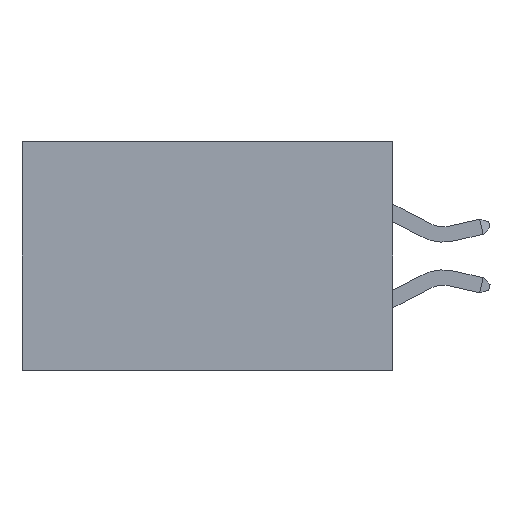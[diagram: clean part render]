
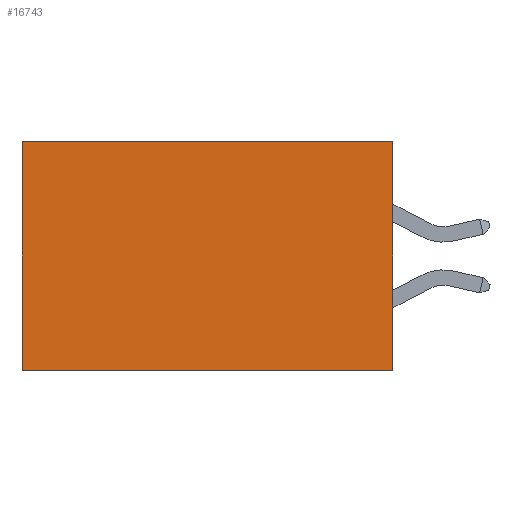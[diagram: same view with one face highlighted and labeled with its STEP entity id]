
A CAD part, left-side view. The second image highlights one B-rep face of the part: STEP entity #16743.
In plain terms, the highlighted planar face has unit normal (-1, 0, 0).
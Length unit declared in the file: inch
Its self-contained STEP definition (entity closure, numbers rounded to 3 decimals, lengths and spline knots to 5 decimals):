
#55 = EDGE_CURVE ( 'NONE', #21798, #2846, #15903, .T. ) ;
#849 = CARTESIAN_POINT ( 'NONE',  ( 0.2875, 0., 0. ) ) ;
#1491 = DIRECTION ( 'NONE',  ( 0., 1., 0. ) ) ;
#2163 = LINE ( 'NONE', #11812, #12779 ) ;
#2846 = VERTEX_POINT ( 'NONE', #5089 ) ;
#2888 = ORIENTED_EDGE ( 'NONE', *, *, #18372, .T. ) ;
#4056 = CARTESIAN_POINT ( 'NONE',  ( 0.2875, 0., -0.37 ) ) ;
#4487 = EDGE_CURVE ( 'NONE', #7276, #12531, #11634, .T. ) ;
#4743 = CARTESIAN_POINT ( 'NONE',  ( 0.2875, 0., -0.37 ) ) ;
#5089 = CARTESIAN_POINT ( 'NONE',  ( 0.2875, 0.6, -0.37 ) ) ;
#5370 = DIRECTION ( 'NONE',  ( 1., 0., 0. ) ) ;
#7140 = CARTESIAN_POINT ( 'NONE',  ( 0.2875, 0., 0. ) ) ;
#7276 = VERTEX_POINT ( 'NONE', #20583 ) ;
#7983 = CARTESIAN_POINT ( 'NONE',  ( 0.2875, 0.6, 0. ) ) ;
#8122 = FACE_OUTER_BOUND ( 'NONE', #11953, .T. ) ;
#8790 = DIRECTION ( 'NONE',  ( 0., 0., -1. ) ) ;
#10014 = EDGE_CURVE ( 'NONE', #12531, #2846, #17494, .T. ) ;
#10182 = DIRECTION ( 'NONE',  ( 0., 1., 0. ) ) ;
#11108 = VECTOR ( 'NONE', #18869, 39.37008 ) ;
#11634 = LINE ( 'NONE', #849, #11108 ) ;
#11812 = CARTESIAN_POINT ( 'NONE',  ( 0.2875, 0., 0. ) ) ;
#11953 = EDGE_LOOP ( 'NONE', ( #12798, #17719, #13572, #2888 ) ) ;
#12531 = VERTEX_POINT ( 'NONE', #4056 ) ;
#12779 = VECTOR ( 'NONE', #10182, 39.37008 ) ;
#12798 = ORIENTED_EDGE ( 'NONE', *, *, #55, .T. ) ;
#12972 = VECTOR ( 'NONE', #15302, 39.37008 ) ;
#13572 = ORIENTED_EDGE ( 'NONE', *, *, #4487, .F. ) ;
#14070 = AXIS2_PLACEMENT_3D ( 'NONE', #7140, #5370, #8790 ) ;
#15302 = DIRECTION ( 'NONE',  ( 0., 0., -1. ) ) ;
#15780 = PLANE ( 'NONE',  #14070 ) ;
#15903 = LINE ( 'NONE', #16858, #12972 ) ;
#16432 = VECTOR ( 'NONE', #1491, 39.37008 ) ;
#16743 = ADVANCED_FACE ( 'NONE', ( #8122 ), #15780, .F. ) ;
#16858 = CARTESIAN_POINT ( 'NONE',  ( 0.2875, 0.6, 0. ) ) ;
#17494 = LINE ( 'NONE', #4743, #16432 ) ;
#17719 = ORIENTED_EDGE ( 'NONE', *, *, #10014, .F. ) ;
#18372 = EDGE_CURVE ( 'NONE', #7276, #21798, #2163, .T. ) ;
#18869 = DIRECTION ( 'NONE',  ( 0., 0., -1. ) ) ;
#20583 = CARTESIAN_POINT ( 'NONE',  ( 0.2875, 0., 0. ) ) ;
#21798 = VERTEX_POINT ( 'NONE', #7983 ) ;
